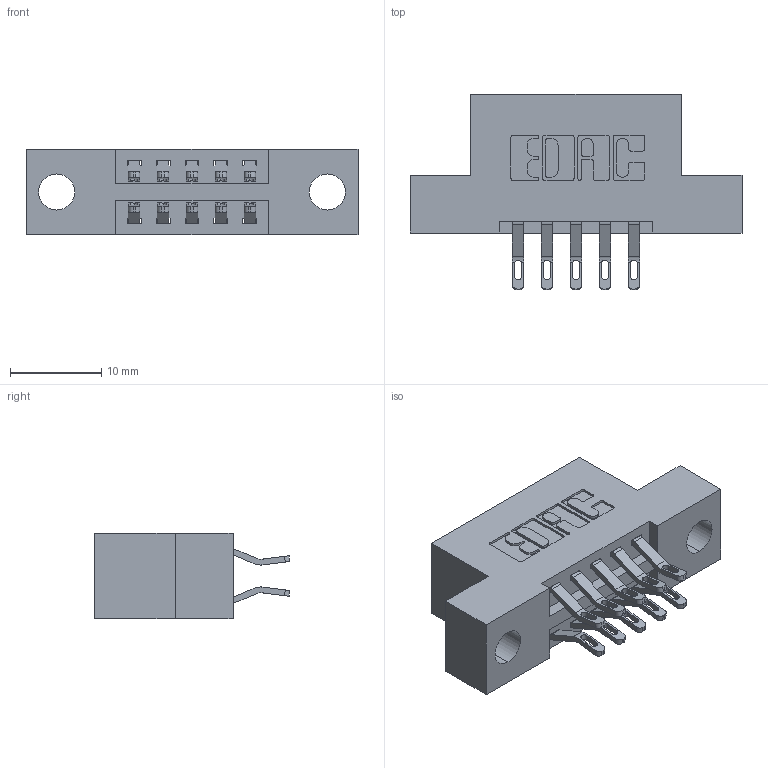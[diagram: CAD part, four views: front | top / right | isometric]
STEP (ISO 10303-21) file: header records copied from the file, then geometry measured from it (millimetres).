
FILE_DESCRIPTION (( 'STEP AP203' ), '1' );
FILE_NAME ('346-010-555-204.STEP', '2022-05-17T17:46:58', ( '' ), ( '' ), 'SwSTEP 2.0', 'SolidWorks 2020', '' );
FILE_SCHEMA (( 'CONFIG_CONTROL_DESIGN' ));
Length unit declared in the file: inch
Products named in the file (3): 346-010-555-204; 346 Part_Flush Mounting Lugs - 0.156 Dia-TH; 345-292-001_555 Tail
Assembly tree (11 placements, depth 2):
  346-010-555-204
    346 Part_Flush Mounting Lugs - 0.156 Dia-TH
    345-292-001_555 Tail  x10
Bounding box: 36.45 x 21.46 x 9.4 mm (x, y, z)
Volume: 3189.9 mm3; surface area: 3754.5 mm2
Topology: 11 solids, 11 shells, 716 faces, 2195 edges, 1462 vertices
Faces by surface type: plane 420, cylinder 296
Entity records: 8989 total; most frequent: CARTESIAN_POINT 1572, ORIENTED_EDGE 1474, DIRECTION 1405, EDGE_CURVE 737, LINE 565, VECTOR 565, VERTEX_POINT 490, AXIS2_PLACEMENT_3D 420
